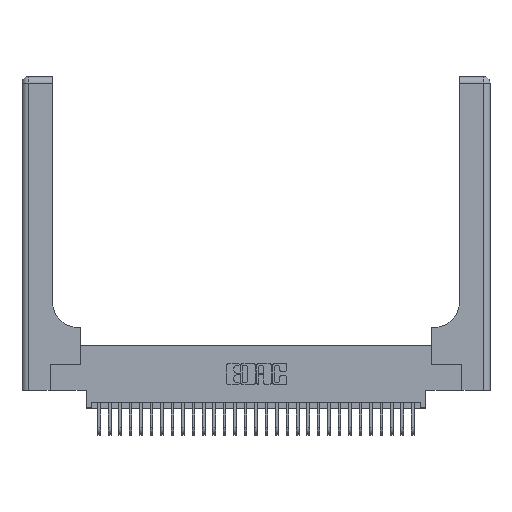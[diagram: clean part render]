
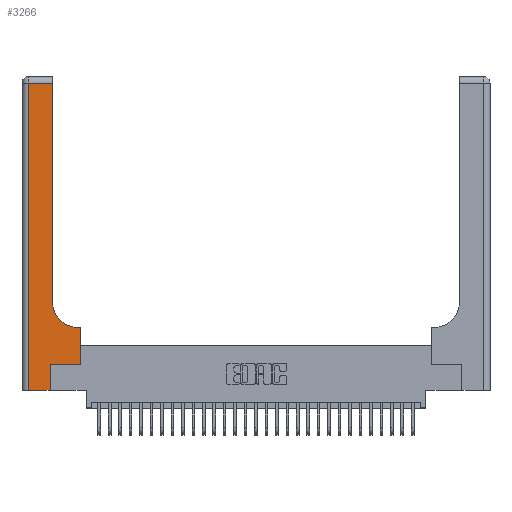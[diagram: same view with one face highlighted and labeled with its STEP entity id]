
A CAD part, top view. The second image highlights one B-rep face of the part: STEP entity #3266.
In plain terms, the highlighted planar face has unit normal (0, 0, 1).
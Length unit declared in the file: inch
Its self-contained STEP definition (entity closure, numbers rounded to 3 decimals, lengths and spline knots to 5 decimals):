
#57 = FACE_OUTER_BOUND ( 'NONE', #27947, .T. ) ;
#715 = CARTESIAN_POINT ( 'NONE',  ( 0.269, 0., 0.37 ) ) ;
#1319 = DIRECTION ( 'NONE',  ( -1., 0., 0. ) ) ;
#1404 = EDGE_CURVE ( 'NONE', #3305, #12321, #25747, .T. ) ;
#2189 = EDGE_CURVE ( 'NONE', #10393, #17532, #10804, .T. ) ;
#3266 = ADVANCED_FACE ( 'NONE', ( #57 ), #20900, .F. ) ;
#3305 = VERTEX_POINT ( 'NONE', #9433 ) ;
#3878 = LINE ( 'NONE', #20357, #15546 ) ;
#4042 = EDGE_CURVE ( 'NONE', #18115, #18911, #11684, .T. ) ;
#4576 = ORIENTED_EDGE ( 'NONE', *, *, #16310, .T. ) ;
#4626 = CARTESIAN_POINT ( 'NONE',  ( 0.5585, 0.25, 0.37 ) ) ;
#4629 = CARTESIAN_POINT ( 'NONE',  ( 0., 3., 0.37 ) ) ;
#4706 = AXIS2_PLACEMENT_3D ( 'NONE', #7943, #24166, #10268 ) ;
#5390 = VECTOR ( 'NONE', #11647, 39.37008 ) ;
#5398 = EDGE_CURVE ( 'NONE', #24714, #21338, #19231, .T. ) ;
#6415 = EDGE_CURVE ( 'NONE', #21338, #29592, #3878, .T. ) ;
#6861 = LINE ( 'NONE', #4626, #5390 ) ;
#6876 = DIRECTION ( 'NONE',  ( 1., 0., 0. ) ) ;
#6880 = VECTOR ( 'NONE', #14146, 39.37008 ) ;
#6980 = DIRECTION ( 'NONE',  ( 0., 0., -1. ) ) ;
#7231 = LINE ( 'NONE', #715, #25762 ) ;
#7630 = ORIENTED_EDGE ( 'NONE', *, *, #1404, .T. ) ;
#7943 = CARTESIAN_POINT ( 'NONE',  ( 0.5415, 0.85, 0.37 ) ) ;
#9433 = CARTESIAN_POINT ( 'NONE',  ( 0.06, 0., 0.37 ) ) ;
#10185 = CARTESIAN_POINT ( 'NONE',  ( 0.269, 0.25, 0.37 ) ) ;
#10268 = DIRECTION ( 'NONE',  ( 1., 0., 0. ) ) ;
#10393 = VERTEX_POINT ( 'NONE', #11026 ) ;
#10804 = LINE ( 'NONE', #10185, #17711 ) ;
#11026 = CARTESIAN_POINT ( 'NONE',  ( 0.269, 0.25, 0.37 ) ) ;
#11351 = EDGE_CURVE ( 'NONE', #18911, #24714, #26066, .T. ) ;
#11647 = DIRECTION ( 'NONE',  ( 0., 1., 0. ) ) ;
#11684 = LINE ( 'NONE', #24551, #23291 ) ;
#12321 = VERTEX_POINT ( 'NONE', #15895 ) ;
#12455 = LINE ( 'NONE', #15293, #24789 ) ;
#12550 = ORIENTED_EDGE ( 'NONE', *, *, #5398, .T. ) ;
#13398 = VECTOR ( 'NONE', #6876, 39.37008 ) ;
#14146 = DIRECTION ( 'NONE',  ( 0., 1., 0. ) ) ;
#14170 = CARTESIAN_POINT ( 'NONE',  ( 0.5585, 0.6, 0.37 ) ) ;
#15293 = CARTESIAN_POINT ( 'NONE',  ( 0.06, 3., 0.37 ) ) ;
#15415 = ORIENTED_EDGE ( 'NONE', *, *, #27037, .T. ) ;
#15546 = VECTOR ( 'NONE', #18023, 39.37008 ) ;
#15697 = ORIENTED_EDGE ( 'NONE', *, *, #6415, .T. ) ;
#15895 = CARTESIAN_POINT ( 'NONE',  ( 0.269, 0., 0.37 ) ) ;
#15902 = CARTESIAN_POINT ( 'NONE',  ( 0.2915, 2.94, 0.37 ) ) ;
#16310 = EDGE_CURVE ( 'NONE', #12321, #10393, #7231, .T. ) ;
#17459 = CARTESIAN_POINT ( 'NONE',  ( 0.5415, 0.6, 0.37 ) ) ;
#17532 = VERTEX_POINT ( 'NONE', #28278 ) ;
#17610 = DIRECTION ( 'NONE',  ( 0., -1., 0. ) ) ;
#17711 = VECTOR ( 'NONE', #26417, 39.37008 ) ;
#18023 = DIRECTION ( 'NONE',  ( -1., 0., 0. ) ) ;
#18115 = VERTEX_POINT ( 'NONE', #14170 ) ;
#18911 = VERTEX_POINT ( 'NONE', #17459 ) ;
#19231 = LINE ( 'NONE', #27816, #6880 ) ;
#19916 = ORIENTED_EDGE ( 'NONE', *, *, #24728, .T. ) ;
#20357 = CARTESIAN_POINT ( 'NONE',  ( 0., 2.94, 0.37 ) ) ;
#20595 = AXIS2_PLACEMENT_3D ( 'NONE', #4629, #6980, #23207 ) ;
#20900 = PLANE ( 'NONE',  #20595 ) ;
#21338 = VERTEX_POINT ( 'NONE', #15902 ) ;
#23089 = CARTESIAN_POINT ( 'NONE',  ( 0., 0., 0.37 ) ) ;
#23207 = DIRECTION ( 'NONE',  ( -1., 0., 0. ) ) ;
#23270 = ORIENTED_EDGE ( 'NONE', *, *, #11351, .T. ) ;
#23291 = VECTOR ( 'NONE', #1319, 39.37008 ) ;
#24071 = DIRECTION ( 'NONE',  ( 0., 1., 0. ) ) ;
#24166 = DIRECTION ( 'NONE',  ( 0., 0., -1. ) ) ;
#24551 = CARTESIAN_POINT ( 'NONE',  ( 0.2915, 0.6, 0.37 ) ) ;
#24714 = VERTEX_POINT ( 'NONE', #29141 ) ;
#24728 = EDGE_CURVE ( 'NONE', #29592, #3305, #12455, .T. ) ;
#24789 = VECTOR ( 'NONE', #17610, 39.37008 ) ;
#25747 = LINE ( 'NONE', #23089, #13398 ) ;
#25762 = VECTOR ( 'NONE', #24071, 39.37008 ) ;
#26066 = CIRCLE ( 'NONE', #4706, 0.25 ) ;
#26417 = DIRECTION ( 'NONE',  ( 1., 0., 0. ) ) ;
#27037 = EDGE_CURVE ( 'NONE', #17532, #18115, #6861, .T. ) ;
#27816 = CARTESIAN_POINT ( 'NONE',  ( 0.2915, 3., 0.37 ) ) ;
#27947 = EDGE_LOOP ( 'NONE', ( #12550, #15697, #19916, #7630, #4576, #30172, #15415, #28642, #23270 ) ) ;
#28278 = CARTESIAN_POINT ( 'NONE',  ( 0.5585, 0.25, 0.37 ) ) ;
#28642 = ORIENTED_EDGE ( 'NONE', *, *, #4042, .T. ) ;
#28871 = CARTESIAN_POINT ( 'NONE',  ( 0.06, 2.94, 0.37 ) ) ;
#29141 = CARTESIAN_POINT ( 'NONE',  ( 0.2915, 0.85, 0.37 ) ) ;
#29592 = VERTEX_POINT ( 'NONE', #28871 ) ;
#30172 = ORIENTED_EDGE ( 'NONE', *, *, #2189, .T. ) ;
